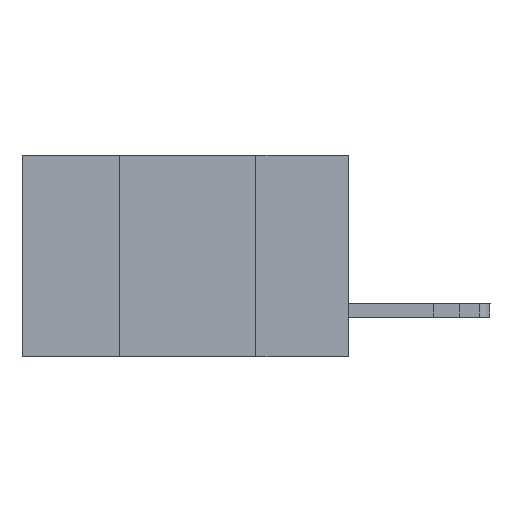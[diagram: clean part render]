
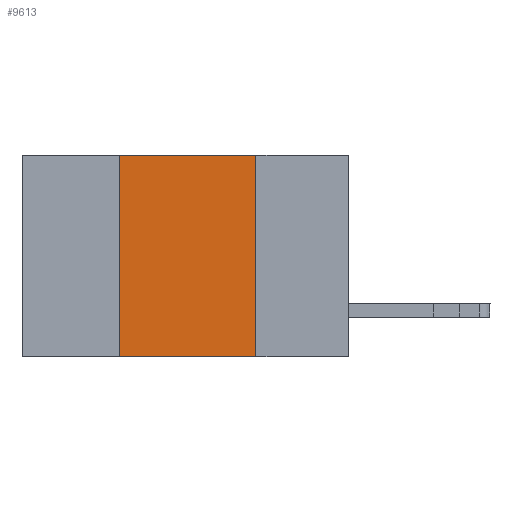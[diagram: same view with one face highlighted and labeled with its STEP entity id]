
A CAD part, left-side view. The second image highlights one B-rep face of the part: STEP entity #9613.
In plain terms, the highlighted planar face has unit normal (-1, 0, 0).
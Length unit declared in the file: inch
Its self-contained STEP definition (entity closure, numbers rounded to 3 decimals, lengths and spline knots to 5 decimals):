
#1075 = CARTESIAN_POINT ( 'NONE',  ( 0., 0.6, -0.37 ) ) ;
#1409 = CARTESIAN_POINT ( 'NONE',  ( 0., 0.6, 0. ) ) ;
#1728 = EDGE_CURVE ( 'NONE', #10261, #16815, #10849, .T. ) ;
#2423 = VERTEX_POINT ( 'NONE', #10266 ) ;
#3281 = VECTOR ( 'NONE', #14651, 39.37008 ) ;
#3864 = LINE ( 'NONE', #5681, #14666 ) ;
#3915 = CARTESIAN_POINT ( 'NONE',  ( 0., 0.17, 0. ) ) ;
#4578 = ORIENTED_EDGE ( 'NONE', *, *, #7142, .F. ) ;
#4727 = CARTESIAN_POINT ( 'NONE',  ( 0., 0.42, 0. ) ) ;
#5394 = ORIENTED_EDGE ( 'NONE', *, *, #15545, .F. ) ;
#5564 = VECTOR ( 'NONE', #16962, 39.37008 ) ;
#5681 = CARTESIAN_POINT ( 'NONE',  ( 0., 0.17, -0.37 ) ) ;
#6875 = VECTOR ( 'NONE', #9346, 39.37008 ) ;
#7142 = EDGE_CURVE ( 'NONE', #16815, #19256, #3864, .T. ) ;
#7882 = PLANE ( 'NONE',  #12087 ) ;
#9124 = ORIENTED_EDGE ( 'NONE', *, *, #18129, .T. ) ;
#9346 = DIRECTION ( 'NONE',  ( 0., -1., 0. ) ) ;
#9613 = ADVANCED_FACE ( 'NONE', ( #10958 ), #7882, .F. ) ;
#10261 = VERTEX_POINT ( 'NONE', #4727 ) ;
#10266 = CARTESIAN_POINT ( 'NONE',  ( 0., 0.42, -0.37 ) ) ;
#10483 = LINE ( 'NONE', #1075, #6875 ) ;
#10510 = CARTESIAN_POINT ( 'NONE',  ( 0., 0.6, 0. ) ) ;
#10849 = LINE ( 'NONE', #10510, #5564 ) ;
#10958 = FACE_OUTER_BOUND ( 'NONE', #17110, .T. ) ;
#12087 = AXIS2_PLACEMENT_3D ( 'NONE', #1409, #14333, #12559 ) ;
#12559 = DIRECTION ( 'NONE',  ( 0., 0., -1. ) ) ;
#13178 = LINE ( 'NONE', #19429, #3281 ) ;
#13644 = CARTESIAN_POINT ( 'NONE',  ( 0., 0.17, -0.37 ) ) ;
#14333 = DIRECTION ( 'NONE',  ( 1., 0., 0. ) ) ;
#14651 = DIRECTION ( 'NONE',  ( 0., 0., 1. ) ) ;
#14666 = VECTOR ( 'NONE', #18458, 39.37008 ) ;
#15545 = EDGE_CURVE ( 'NONE', #2423, #10261, #13178, .T. ) ;
#16815 = VERTEX_POINT ( 'NONE', #3915 ) ;
#16962 = DIRECTION ( 'NONE',  ( 0., -1., 0. ) ) ;
#17110 = EDGE_LOOP ( 'NONE', ( #4578, #18033, #5394, #9124 ) ) ;
#18033 = ORIENTED_EDGE ( 'NONE', *, *, #1728, .F. ) ;
#18129 = EDGE_CURVE ( 'NONE', #2423, #19256, #10483, .T. ) ;
#18458 = DIRECTION ( 'NONE',  ( 0., 0., -1. ) ) ;
#19256 = VERTEX_POINT ( 'NONE', #13644 ) ;
#19429 = CARTESIAN_POINT ( 'NONE',  ( 0., 0.42, -0.37 ) ) ;
